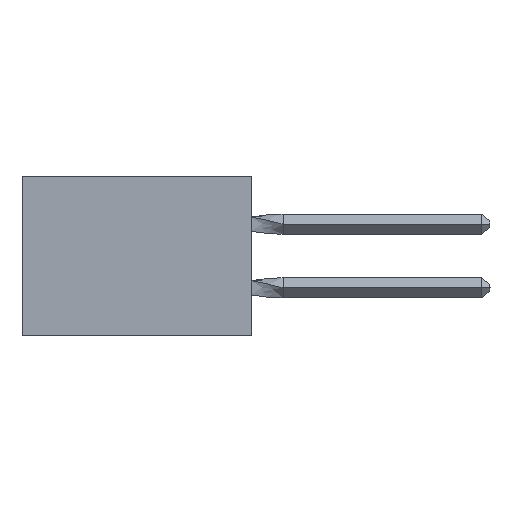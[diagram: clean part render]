
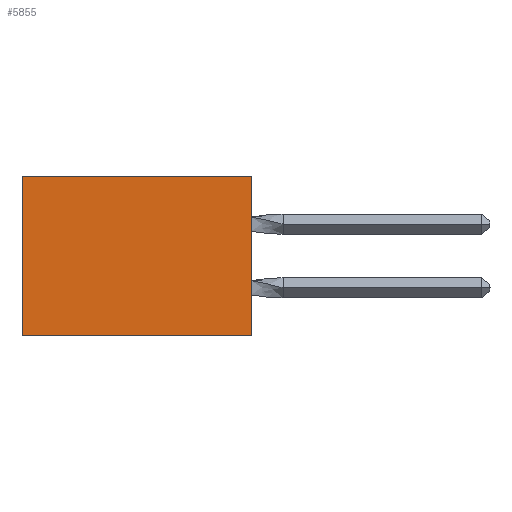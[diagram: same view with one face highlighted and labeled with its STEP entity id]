
A CAD part, left-side view. The second image highlights one B-rep face of the part: STEP entity #5855.
In plain terms, the highlighted planar face has unit normal (-1, 0, 0).
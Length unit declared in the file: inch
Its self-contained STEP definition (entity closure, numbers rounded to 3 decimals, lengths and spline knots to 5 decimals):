
#104 = DIRECTION ( 'NONE',  ( 0., 0., -1. ) ) ;
#468 = EDGE_CURVE ( 'NONE', #15548, #984, #3598, .T. ) ;
#777 = DIRECTION ( 'NONE',  ( 0., 1., 0. ) ) ;
#976 = EDGE_CURVE ( 'NONE', #13081, #15548, #4001, .T. ) ;
#984 = VERTEX_POINT ( 'NONE', #8565 ) ;
#1016 = LINE ( 'NONE', #5657, #6805 ) ;
#1903 = FACE_OUTER_BOUND ( 'NONE', #10220, .T. ) ;
#2963 = PLANE ( 'NONE',  #10711 ) ;
#3598 = LINE ( 'NONE', #5133, #13750 ) ;
#4001 = LINE ( 'NONE', #7328, #13927 ) ;
#5133 = CARTESIAN_POINT ( 'NONE',  ( 0.305, 0., -0.5 ) ) ;
#5220 = ORIENTED_EDGE ( 'NONE', *, *, #468, .F. ) ;
#5657 = CARTESIAN_POINT ( 'NONE',  ( 0.305, 0., 0. ) ) ;
#5855 = ADVANCED_FACE ( 'NONE', ( #1903 ), #2963, .F. ) ;
#6805 = VECTOR ( 'NONE', #777, 39.37008 ) ;
#7328 = CARTESIAN_POINT ( 'NONE',  ( 0.305, 0., -0.5 ) ) ;
#7400 = EDGE_CURVE ( 'NONE', #11871, #984, #15147, .T. ) ;
#7855 = DIRECTION ( 'NONE',  ( 1., 0., 0. ) ) ;
#8077 = ORIENTED_EDGE ( 'NONE', *, *, #7400, .T. ) ;
#8565 = CARTESIAN_POINT ( 'NONE',  ( 0.305, 0.72, -0.5 ) ) ;
#9694 = CARTESIAN_POINT ( 'NONE',  ( 0.305, 0., -0.5 ) ) ;
#10220 = EDGE_LOOP ( 'NONE', ( #8077, #5220, #14156, #11749 ) ) ;
#10711 = AXIS2_PLACEMENT_3D ( 'NONE', #11433, #7855, #15067 ) ;
#11433 = CARTESIAN_POINT ( 'NONE',  ( 0.305, 0., -0.5 ) ) ;
#11749 = ORIENTED_EDGE ( 'NONE', *, *, #12058, .T. ) ;
#11871 = VERTEX_POINT ( 'NONE', #14754 ) ;
#12058 = EDGE_CURVE ( 'NONE', #13081, #11871, #1016, .T. ) ;
#12856 = VECTOR ( 'NONE', #13937, 39.37008 ) ;
#13081 = VERTEX_POINT ( 'NONE', #14521 ) ;
#13750 = VECTOR ( 'NONE', #14877, 39.37008 ) ;
#13886 = CARTESIAN_POINT ( 'NONE',  ( 0.305, 0.72, -0.5 ) ) ;
#13927 = VECTOR ( 'NONE', #104, 39.37008 ) ;
#13937 = DIRECTION ( 'NONE',  ( 0., 0., -1. ) ) ;
#14156 = ORIENTED_EDGE ( 'NONE', *, *, #976, .F. ) ;
#14521 = CARTESIAN_POINT ( 'NONE',  ( 0.305, 0., 0. ) ) ;
#14754 = CARTESIAN_POINT ( 'NONE',  ( 0.305, 0.72, 0. ) ) ;
#14877 = DIRECTION ( 'NONE',  ( 0., 1., 0. ) ) ;
#15067 = DIRECTION ( 'NONE',  ( 0., 0., -1. ) ) ;
#15147 = LINE ( 'NONE', #13886, #12856 ) ;
#15548 = VERTEX_POINT ( 'NONE', #9694 ) ;
